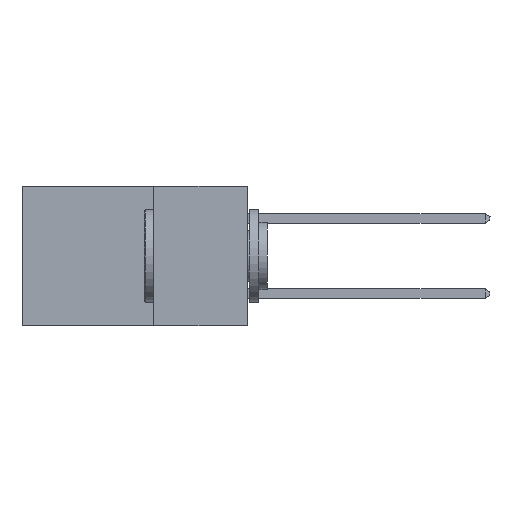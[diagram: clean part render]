
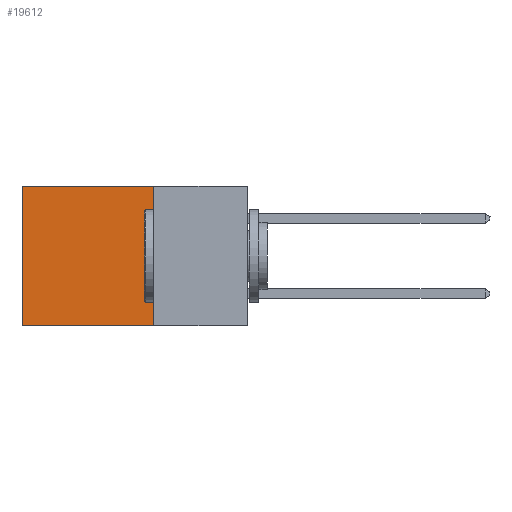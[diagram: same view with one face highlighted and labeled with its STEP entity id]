
A CAD part, left-side view. The second image highlights one B-rep face of the part: STEP entity #19612.
In plain terms, the highlighted planar face has unit normal (-1, 0, 0).
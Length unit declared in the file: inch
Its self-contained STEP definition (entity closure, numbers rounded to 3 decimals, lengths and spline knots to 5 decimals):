
#404 = EDGE_CURVE ( 'NONE', #4445, #5749, #22632, .T. ) ;
#718 = DIRECTION ( 'NONE',  ( 0., 1., 0. ) ) ;
#1613 = DIRECTION ( 'NONE',  ( 0., 0., -1. ) ) ;
#2207 = VECTOR ( 'NONE', #718, 39.37008 ) ;
#2271 = DIRECTION ( 'NONE',  ( 0., 0., -1. ) ) ;
#2366 = CARTESIAN_POINT ( 'NONE',  ( 0.298, 0.25, 0. ) ) ;
#3195 = AXIS2_PLACEMENT_3D ( 'NONE', #12082, #14165, #1613 ) ;
#3219 = EDGE_CURVE ( 'NONE', #25665, #5749, #9262, .T. ) ;
#4445 = VERTEX_POINT ( 'NONE', #23624 ) ;
#5749 = VERTEX_POINT ( 'NONE', #11966 ) ;
#7448 = EDGE_CURVE ( 'NONE', #9574, #25665, #15714, .T. ) ;
#8261 = VECTOR ( 'NONE', #2271, 39.37008 ) ;
#8422 = ORIENTED_EDGE ( 'NONE', *, *, #3219, .F. ) ;
#9262 = LINE ( 'NONE', #18727, #14142 ) ;
#9371 = DIRECTION ( 'NONE',  ( 0., 1., 0. ) ) ;
#9574 = VERTEX_POINT ( 'NONE', #18371 ) ;
#9990 = EDGE_CURVE ( 'NONE', #9574, #4445, #18170, .T. ) ;
#11966 = CARTESIAN_POINT ( 'NONE',  ( 0.298, 0.6, -0.37 ) ) ;
#11993 = EDGE_LOOP ( 'NONE', ( #12249, #8422, #17966, #26120 ) ) ;
#12082 = CARTESIAN_POINT ( 'NONE',  ( 0.298, 0.25, 0. ) ) ;
#12249 = ORIENTED_EDGE ( 'NONE', *, *, #404, .T. ) ;
#13271 = CARTESIAN_POINT ( 'NONE',  ( 0.298, 0.25, 0. ) ) ;
#14142 = VECTOR ( 'NONE', #9371, 39.37008 ) ;
#14165 = DIRECTION ( 'NONE',  ( 1., 0., 0. ) ) ;
#15714 = LINE ( 'NONE', #2366, #8261 ) ;
#17966 = ORIENTED_EDGE ( 'NONE', *, *, #7448, .F. ) ;
#18170 = LINE ( 'NONE', #13271, #2207 ) ;
#18371 = CARTESIAN_POINT ( 'NONE',  ( 0.298, 0.25, 0. ) ) ;
#18727 = CARTESIAN_POINT ( 'NONE',  ( 0.298, 0.25, -0.37 ) ) ;
#19612 = ADVANCED_FACE ( 'NONE', ( #25411 ), #24371, .F. ) ;
#22632 = LINE ( 'NONE', #25130, #26663 ) ;
#23624 = CARTESIAN_POINT ( 'NONE',  ( 0.298, 0.6, 0. ) ) ;
#24258 = CARTESIAN_POINT ( 'NONE',  ( 0.298, 0.25, -0.37 ) ) ;
#24371 = PLANE ( 'NONE',  #3195 ) ;
#25130 = CARTESIAN_POINT ( 'NONE',  ( 0.298, 0.6, 0. ) ) ;
#25411 = FACE_OUTER_BOUND ( 'NONE', #11993, .T. ) ;
#25665 = VERTEX_POINT ( 'NONE', #24258 ) ;
#26120 = ORIENTED_EDGE ( 'NONE', *, *, #9990, .T. ) ;
#26400 = DIRECTION ( 'NONE',  ( 0., 0., -1. ) ) ;
#26663 = VECTOR ( 'NONE', #26400, 39.37008 ) ;
